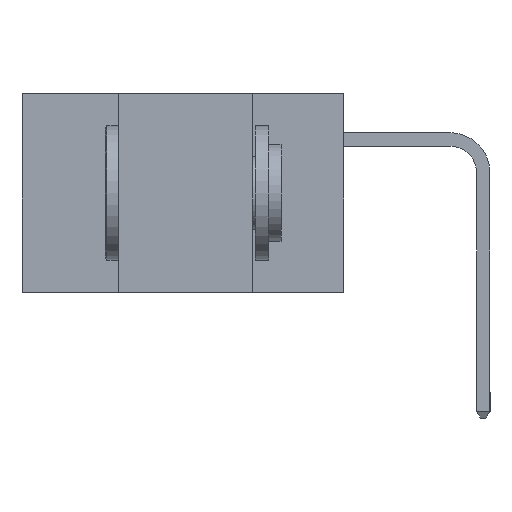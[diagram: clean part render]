
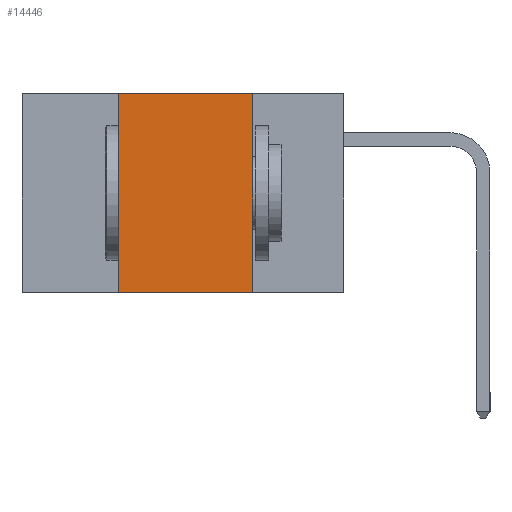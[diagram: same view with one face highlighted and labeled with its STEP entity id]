
A CAD part, left-side view. The second image highlights one B-rep face of the part: STEP entity #14446.
In plain terms, the highlighted planar face has unit normal (-1, 0, 0).
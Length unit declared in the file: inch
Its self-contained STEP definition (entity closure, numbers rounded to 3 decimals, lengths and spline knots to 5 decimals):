
#1778 = FACE_OUTER_BOUND ( 'NONE', #17741, .T. ) ;
#1975 = CARTESIAN_POINT ( 'NONE',  ( 0., 0.17, -0.37 ) ) ;
#2598 = AXIS2_PLACEMENT_3D ( 'NONE', #23355, #15424, #3420 ) ;
#3420 = DIRECTION ( 'NONE',  ( 0., 0., -1. ) ) ;
#4070 = CARTESIAN_POINT ( 'NONE',  ( 0., 0.42, -0.37 ) ) ;
#4081 = EDGE_CURVE ( 'NONE', #16609, #22402, #12667, .T. ) ;
#5189 = CARTESIAN_POINT ( 'NONE',  ( 0., 0.42, 0. ) ) ;
#5402 = EDGE_CURVE ( 'NONE', #16609, #19099, #25928, .T. ) ;
#6247 = CARTESIAN_POINT ( 'NONE',  ( 0., 0.17, 0. ) ) ;
#7244 = CARTESIAN_POINT ( 'NONE',  ( 0., 0.6, -0.37 ) ) ;
#7737 = ORIENTED_EDGE ( 'NONE', *, *, #22624, .F. ) ;
#9154 = CARTESIAN_POINT ( 'NONE',  ( 0., 0.17, 0. ) ) ;
#9367 = LINE ( 'NONE', #10754, #19446 ) ;
#9433 = EDGE_CURVE ( 'NONE', #22734, #22402, #24402, .T. ) ;
#10754 = CARTESIAN_POINT ( 'NONE',  ( 0., 0.6, 0. ) ) ;
#12399 = DIRECTION ( 'NONE',  ( 0., -1., 0. ) ) ;
#12607 = ORIENTED_EDGE ( 'NONE', *, *, #4081, .T. ) ;
#12667 = LINE ( 'NONE', #7244, #23273 ) ;
#13043 = ORIENTED_EDGE ( 'NONE', *, *, #9433, .F. ) ;
#13156 = VECTOR ( 'NONE', #14300, 39.37008 ) ;
#14300 = DIRECTION ( 'NONE',  ( 0., 0., -1. ) ) ;
#14446 = ADVANCED_FACE ( 'NONE', ( #1778 ), #25306, .F. ) ;
#15384 = VECTOR ( 'NONE', #19931, 39.37008 ) ;
#15424 = DIRECTION ( 'NONE',  ( 1., 0., 0. ) ) ;
#16609 = VERTEX_POINT ( 'NONE', #4070 ) ;
#17741 = EDGE_LOOP ( 'NONE', ( #13043, #7737, #22011, #12607 ) ) ;
#18764 = CARTESIAN_POINT ( 'NONE',  ( 0., 0.42, 0. ) ) ;
#18855 = DIRECTION ( 'NONE',  ( 0., -1., 0. ) ) ;
#19099 = VERTEX_POINT ( 'NONE', #5189 ) ;
#19446 = VECTOR ( 'NONE', #18855, 39.37008 ) ;
#19931 = DIRECTION ( 'NONE',  ( 0., 0., 1. ) ) ;
#22011 = ORIENTED_EDGE ( 'NONE', *, *, #5402, .F. ) ;
#22402 = VERTEX_POINT ( 'NONE', #1975 ) ;
#22624 = EDGE_CURVE ( 'NONE', #19099, #22734, #9367, .T. ) ;
#22734 = VERTEX_POINT ( 'NONE', #9154 ) ;
#23273 = VECTOR ( 'NONE', #12399, 39.37008 ) ;
#23355 = CARTESIAN_POINT ( 'NONE',  ( 0., 0.6, 0. ) ) ;
#24402 = LINE ( 'NONE', #6247, #13156 ) ;
#25306 = PLANE ( 'NONE',  #2598 ) ;
#25928 = LINE ( 'NONE', #18764, #15384 ) ;
